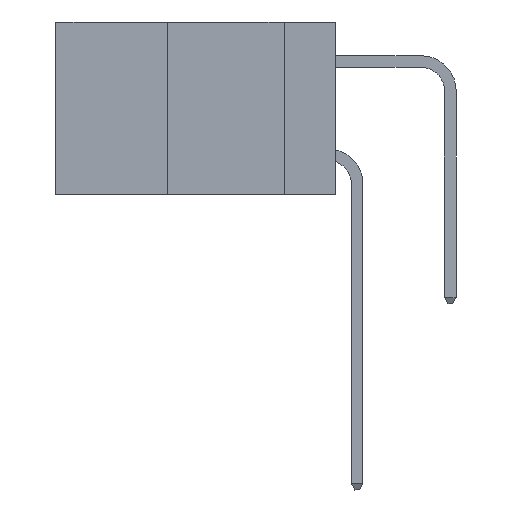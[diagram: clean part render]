
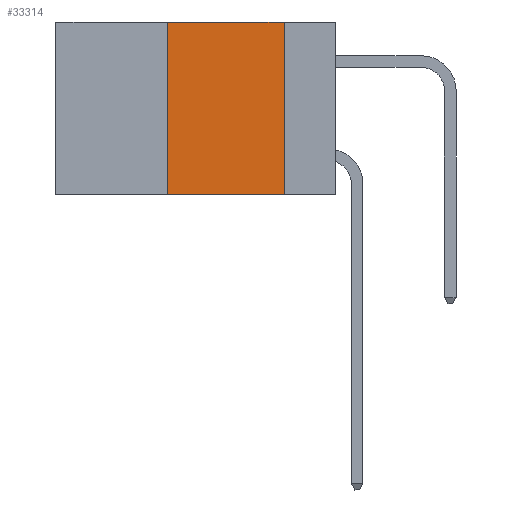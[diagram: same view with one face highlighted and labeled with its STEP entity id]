
A CAD part, left-side view. The second image highlights one B-rep face of the part: STEP entity #33314.
In plain terms, the highlighted planar face has unit normal (-1, 0, 0).
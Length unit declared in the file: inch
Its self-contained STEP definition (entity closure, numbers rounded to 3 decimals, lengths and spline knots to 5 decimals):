
#366 = EDGE_CURVE ( 'NONE', #26643, #20153, #7107, .T. ) ;
#1773 = CARTESIAN_POINT ( 'NONE',  ( 0., 0.11, -0.37 ) ) ;
#2039 = CARTESIAN_POINT ( 'NONE',  ( 0., 0.36, -0.37 ) ) ;
#2432 = ORIENTED_EDGE ( 'NONE', *, *, #366, .T. ) ;
#3112 = DIRECTION ( 'NONE',  ( 0., 0., -1. ) ) ;
#5000 = CARTESIAN_POINT ( 'NONE',  ( 0., 0.6, -0.37 ) ) ;
#7107 = LINE ( 'NONE', #5000, #34648 ) ;
#7150 = VECTOR ( 'NONE', #24890, 39.37008 ) ;
#7153 = FACE_OUTER_BOUND ( 'NONE', #17129, .T. ) ;
#8174 = VERTEX_POINT ( 'NONE', #19935 ) ;
#10450 = DIRECTION ( 'NONE',  ( 1., 0., 0. ) ) ;
#10890 = EDGE_CURVE ( 'NONE', #8174, #20153, #13327, .T. ) ;
#11954 = EDGE_CURVE ( 'NONE', #26643, #17723, #15080, .T. ) ;
#13327 = LINE ( 'NONE', #20882, #36121 ) ;
#15080 = LINE ( 'NONE', #16430, #7150 ) ;
#16430 = CARTESIAN_POINT ( 'NONE',  ( 0., 0.36, 0. ) ) ;
#16547 = CARTESIAN_POINT ( 'NONE',  ( 0., 0.6, 0. ) ) ;
#17129 = EDGE_LOOP ( 'NONE', ( #35630, #24197, #30623, #2432 ) ) ;
#17672 = CARTESIAN_POINT ( 'NONE',  ( 0., 0.6, 0. ) ) ;
#17723 = VERTEX_POINT ( 'NONE', #22869 ) ;
#19935 = CARTESIAN_POINT ( 'NONE',  ( 0., 0.11, 0. ) ) ;
#20153 = VERTEX_POINT ( 'NONE', #1773 ) ;
#20675 = DIRECTION ( 'NONE',  ( 0., -1., 0. ) ) ;
#20882 = CARTESIAN_POINT ( 'NONE',  ( 0., 0.11, 0. ) ) ;
#21872 = EDGE_CURVE ( 'NONE', #17723, #8174, #32392, .T. ) ;
#22869 = CARTESIAN_POINT ( 'NONE',  ( 0., 0.36, 0. ) ) ;
#24197 = ORIENTED_EDGE ( 'NONE', *, *, #21872, .F. ) ;
#24890 = DIRECTION ( 'NONE',  ( 0., 0., 1. ) ) ;
#25857 = DIRECTION ( 'NONE',  ( 0., -1., 0. ) ) ;
#26643 = VERTEX_POINT ( 'NONE', #2039 ) ;
#30623 = ORIENTED_EDGE ( 'NONE', *, *, #11954, .F. ) ;
#31151 = DIRECTION ( 'NONE',  ( 0., 0., -1. ) ) ;
#32392 = LINE ( 'NONE', #17672, #37981 ) ;
#33314 = ADVANCED_FACE ( 'NONE', ( #7153 ), #34285, .F. ) ;
#34285 = PLANE ( 'NONE',  #36026 ) ;
#34648 = VECTOR ( 'NONE', #25857, 39.37008 ) ;
#35630 = ORIENTED_EDGE ( 'NONE', *, *, #10890, .F. ) ;
#36026 = AXIS2_PLACEMENT_3D ( 'NONE', #16547, #10450, #31151 ) ;
#36121 = VECTOR ( 'NONE', #3112, 39.37008 ) ;
#37981 = VECTOR ( 'NONE', #20675, 39.37008 ) ;
